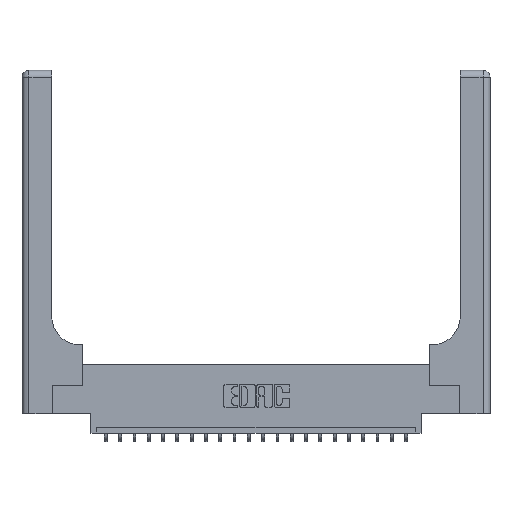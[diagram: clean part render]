
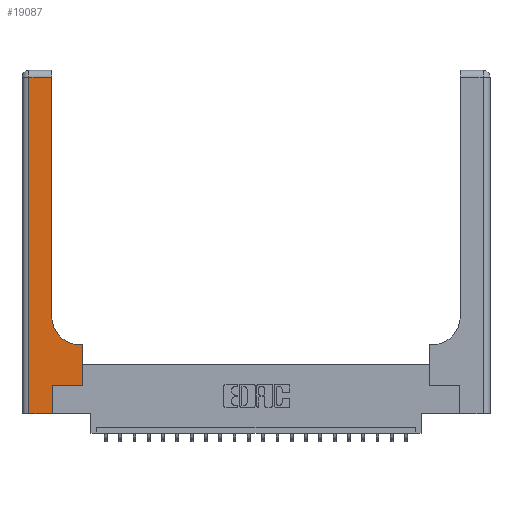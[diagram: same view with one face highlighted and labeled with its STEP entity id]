
A CAD part, top view. The second image highlights one B-rep face of the part: STEP entity #19087.
In plain terms, the highlighted planar face has unit normal (0, 0, 1).
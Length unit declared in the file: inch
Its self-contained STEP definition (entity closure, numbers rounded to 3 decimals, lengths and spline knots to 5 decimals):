
#92 = LINE ( 'NONE', #19891, #5979 ) ;
#236 = ORIENTED_EDGE ( 'NONE', *, *, #2782, .T. ) ;
#519 = EDGE_CURVE ( 'NONE', #20502, #6266, #22091, .T. ) ;
#524 = AXIS2_PLACEMENT_3D ( 'NONE', #13965, #10360, #14187 ) ;
#648 = CARTESIAN_POINT ( 'NONE',  ( 0.26, 2.94, 0.37 ) ) ;
#891 = ORIENTED_EDGE ( 'NONE', *, *, #13115, .T. ) ;
#1221 = DIRECTION ( 'NONE',  ( -1., 0., 0. ) ) ;
#2231 = CARTESIAN_POINT ( 'NONE',  ( 0.528, 0.25, 0.37 ) ) ;
#2366 = DIRECTION ( 'NONE',  ( 0., 1., 0. ) ) ;
#2367 = EDGE_CURVE ( 'NONE', #15626, #5950, #92, .T. ) ;
#2782 = EDGE_CURVE ( 'NONE', #5950, #12464, #8618, .T. ) ;
#3231 = CARTESIAN_POINT ( 'NONE',  ( 0.06, 3., 0.37 ) ) ;
#3320 = CARTESIAN_POINT ( 'NONE',  ( 0.51, 0.85, 0.37 ) ) ;
#3342 = LINE ( 'NONE', #20084, #12904 ) ;
#3933 = VECTOR ( 'NONE', #1221, 39.37008 ) ;
#4083 = CARTESIAN_POINT ( 'NONE',  ( 0.528, 0.6, 0.37 ) ) ;
#4841 = VECTOR ( 'NONE', #19137, 39.37008 ) ;
#4928 = LINE ( 'NONE', #3231, #22186 ) ;
#5851 = VERTEX_POINT ( 'NONE', #17889 ) ;
#5861 = LINE ( 'NONE', #21450, #11320 ) ;
#5950 = VERTEX_POINT ( 'NONE', #12955 ) ;
#5979 = VECTOR ( 'NONE', #16759, 39.37008 ) ;
#6266 = VERTEX_POINT ( 'NONE', #2231 ) ;
#6306 = ORIENTED_EDGE ( 'NONE', *, *, #12624, .T. ) ;
#6543 = ORIENTED_EDGE ( 'NONE', *, *, #519, .T. ) ;
#6735 = DIRECTION ( 'NONE',  ( 1., 0., 0. ) ) ;
#8581 = ORIENTED_EDGE ( 'NONE', *, *, #13245, .T. ) ;
#8618 = CIRCLE ( 'NONE', #21152, 0.25 ) ;
#8698 = CARTESIAN_POINT ( 'NONE',  ( 0.265, 0., 0.37 ) ) ;
#8926 = EDGE_CURVE ( 'NONE', #18655, #20502, #16628, .T. ) ;
#9347 = VECTOR ( 'NONE', #6735, 39.37008 ) ;
#10092 = DIRECTION ( 'NONE',  ( 0., -1., 0. ) ) ;
#10182 = DIRECTION ( 'NONE',  ( 0., 0., -1. ) ) ;
#10360 = DIRECTION ( 'NONE',  ( 0., 0., -1. ) ) ;
#10946 = ORIENTED_EDGE ( 'NONE', *, *, #2367, .T. ) ;
#11320 = VECTOR ( 'NONE', #2366, 39.37008 ) ;
#11441 = CARTESIAN_POINT ( 'NONE',  ( 0.26, 0.85, 0.37 ) ) ;
#12233 = CARTESIAN_POINT ( 'NONE',  ( 0.265, 0.25, 0.37 ) ) ;
#12244 = EDGE_LOOP ( 'NONE', ( #19680, #891, #6306, #8581, #21511, #6543, #14571, #10946, #236 ) ) ;
#12464 = VERTEX_POINT ( 'NONE', #11441 ) ;
#12624 = EDGE_CURVE ( 'NONE', #17741, #5851, #4928, .T. ) ;
#12827 = VECTOR ( 'NONE', #18644, 39.37008 ) ;
#12904 = VECTOR ( 'NONE', #22090, 39.37008 ) ;
#12955 = CARTESIAN_POINT ( 'NONE',  ( 0.51, 0.6, 0.37 ) ) ;
#13115 = EDGE_CURVE ( 'NONE', #13504, #17741, #21974, .T. ) ;
#13245 = EDGE_CURVE ( 'NONE', #5851, #18655, #3342, .T. ) ;
#13504 = VERTEX_POINT ( 'NONE', #648 ) ;
#13965 = CARTESIAN_POINT ( 'NONE',  ( 0., 3., 0.37 ) ) ;
#14187 = DIRECTION ( 'NONE',  ( -1., 0., 0. ) ) ;
#14329 = LINE ( 'NONE', #21036, #4841 ) ;
#14571 = ORIENTED_EDGE ( 'NONE', *, *, #20382, .T. ) ;
#15626 = VERTEX_POINT ( 'NONE', #4083 ) ;
#16628 = LINE ( 'NONE', #18748, #12827 ) ;
#16759 = DIRECTION ( 'NONE',  ( -1., 0., 0. ) ) ;
#17028 = DIRECTION ( 'NONE',  ( 1., 0., 0. ) ) ;
#17050 = CARTESIAN_POINT ( 'NONE',  ( 0., 2.94, 0.37 ) ) ;
#17652 = PLANE ( 'NONE',  #524 ) ;
#17741 = VERTEX_POINT ( 'NONE', #21987 ) ;
#17889 = CARTESIAN_POINT ( 'NONE',  ( 0.06, 0., 0.37 ) ) ;
#18308 = CARTESIAN_POINT ( 'NONE',  ( 0.265, 0.25, 0.37 ) ) ;
#18644 = DIRECTION ( 'NONE',  ( 0., 1., 0. ) ) ;
#18655 = VERTEX_POINT ( 'NONE', #8698 ) ;
#18748 = CARTESIAN_POINT ( 'NONE',  ( 0.265, 0., 0.37 ) ) ;
#18891 = FACE_OUTER_BOUND ( 'NONE', #12244, .T. ) ;
#19087 = ADVANCED_FACE ( 'NONE', ( #18891 ), #17652, .F. ) ;
#19137 = DIRECTION ( 'NONE',  ( 0., 1., 0. ) ) ;
#19680 = ORIENTED_EDGE ( 'NONE', *, *, #19860, .T. ) ;
#19860 = EDGE_CURVE ( 'NONE', #12464, #13504, #14329, .T. ) ;
#19891 = CARTESIAN_POINT ( 'NONE',  ( 0.26, 0.6, 0.37 ) ) ;
#20084 = CARTESIAN_POINT ( 'NONE',  ( 0., 0., 0.37 ) ) ;
#20382 = EDGE_CURVE ( 'NONE', #6266, #15626, #5861, .T. ) ;
#20502 = VERTEX_POINT ( 'NONE', #12233 ) ;
#21036 = CARTESIAN_POINT ( 'NONE',  ( 0.26, 3., 0.37 ) ) ;
#21152 = AXIS2_PLACEMENT_3D ( 'NONE', #3320, #10182, #17028 ) ;
#21450 = CARTESIAN_POINT ( 'NONE',  ( 0.528, 0.25, 0.37 ) ) ;
#21511 = ORIENTED_EDGE ( 'NONE', *, *, #8926, .T. ) ;
#21974 = LINE ( 'NONE', #17050, #3933 ) ;
#21987 = CARTESIAN_POINT ( 'NONE',  ( 0.06, 2.94, 0.37 ) ) ;
#22090 = DIRECTION ( 'NONE',  ( 1., 0., 0. ) ) ;
#22091 = LINE ( 'NONE', #18308, #9347 ) ;
#22186 = VECTOR ( 'NONE', #10092, 39.37008 ) ;
